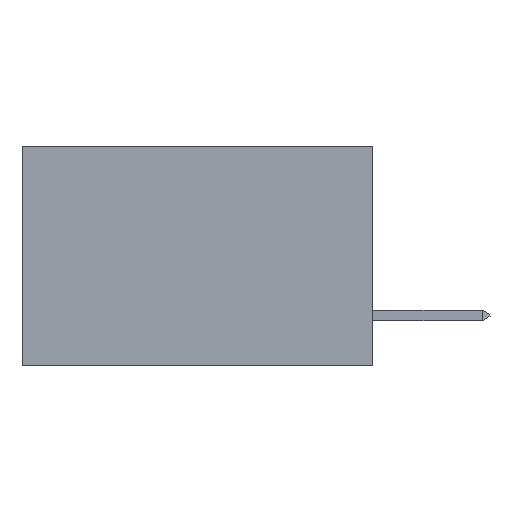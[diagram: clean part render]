
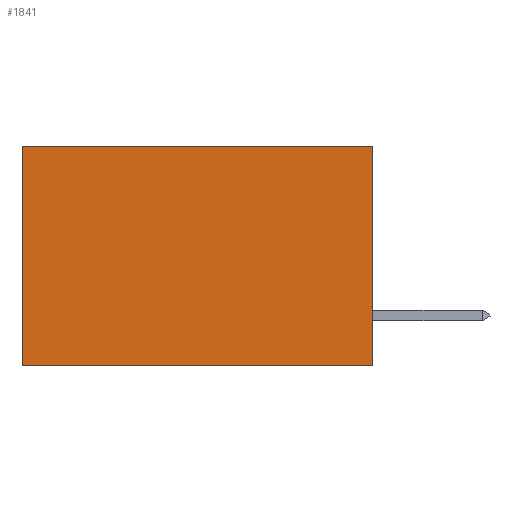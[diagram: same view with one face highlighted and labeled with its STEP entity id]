
A CAD part, left-side view. The second image highlights one B-rep face of the part: STEP entity #1841.
In plain terms, the highlighted planar face has unit normal (-1, 0, 0).
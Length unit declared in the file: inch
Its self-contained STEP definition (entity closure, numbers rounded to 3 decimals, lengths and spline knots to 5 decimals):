
#325 = CARTESIAN_POINT ( 'NONE',  ( 0.277, 0., -0.37 ) ) ;
#426 = DIRECTION ( 'NONE',  ( 0., 0., -1. ) ) ;
#476 = DIRECTION ( 'NONE',  ( 0., 0., -1. ) ) ;
#901 = CARTESIAN_POINT ( 'NONE',  ( 0.277, 0., 0. ) ) ;
#1300 = CARTESIAN_POINT ( 'NONE',  ( 0.277, 0., -0.37 ) ) ;
#1493 = ORIENTED_EDGE ( 'NONE', *, *, #4358, .F. ) ;
#1519 = ORIENTED_EDGE ( 'NONE', *, *, #8306, .T. ) ;
#1591 = DIRECTION ( 'NONE',  ( 0., 1., 0. ) ) ;
#1688 = EDGE_LOOP ( 'NONE', ( #1519, #9335, #1493, #7103 ) ) ;
#1841 = ADVANCED_FACE ( 'NONE', ( #7421 ), #6449, .F. ) ;
#2325 = LINE ( 'NONE', #5713, #2597 ) ;
#2597 = VECTOR ( 'NONE', #5715, 39.37008 ) ;
#3050 = LINE ( 'NONE', #7760, #9464 ) ;
#3521 = VERTEX_POINT ( 'NONE', #9932 ) ;
#3780 = CARTESIAN_POINT ( 'NONE',  ( 0.277, 0., -0.37 ) ) ;
#4102 = VECTOR ( 'NONE', #1591, 39.37008 ) ;
#4358 = EDGE_CURVE ( 'NONE', #6414, #8211, #3050, .T. ) ;
#5250 = VERTEX_POINT ( 'NONE', #8245 ) ;
#5680 = EDGE_CURVE ( 'NONE', #6414, #5250, #2325, .T. ) ;
#5713 = CARTESIAN_POINT ( 'NONE',  ( 0.277, 0., 0. ) ) ;
#5715 = DIRECTION ( 'NONE',  ( 0., 1., 0. ) ) ;
#6219 = DIRECTION ( 'NONE',  ( 0., 0., -1. ) ) ;
#6414 = VERTEX_POINT ( 'NONE', #901 ) ;
#6449 = PLANE ( 'NONE',  #9024 ) ;
#6668 = EDGE_CURVE ( 'NONE', #8211, #3521, #10349, .T. ) ;
#7103 = ORIENTED_EDGE ( 'NONE', *, *, #5680, .T. ) ;
#7421 = FACE_OUTER_BOUND ( 'NONE', #1688, .T. ) ;
#7697 = LINE ( 'NONE', #8221, #7930 ) ;
#7760 = CARTESIAN_POINT ( 'NONE',  ( 0.277, 0., -0.37 ) ) ;
#7930 = VECTOR ( 'NONE', #476, 39.37008 ) ;
#8211 = VERTEX_POINT ( 'NONE', #325 ) ;
#8221 = CARTESIAN_POINT ( 'NONE',  ( 0.277, 0.59, -0.37 ) ) ;
#8245 = CARTESIAN_POINT ( 'NONE',  ( 0.277, 0.59, 0. ) ) ;
#8306 = EDGE_CURVE ( 'NONE', #5250, #3521, #7697, .T. ) ;
#9024 = AXIS2_PLACEMENT_3D ( 'NONE', #3780, #10130, #426 ) ;
#9335 = ORIENTED_EDGE ( 'NONE', *, *, #6668, .F. ) ;
#9464 = VECTOR ( 'NONE', #6219, 39.37008 ) ;
#9932 = CARTESIAN_POINT ( 'NONE',  ( 0.277, 0.59, -0.37 ) ) ;
#10130 = DIRECTION ( 'NONE',  ( 1., 0., 0. ) ) ;
#10349 = LINE ( 'NONE', #1300, #4102 ) ;
